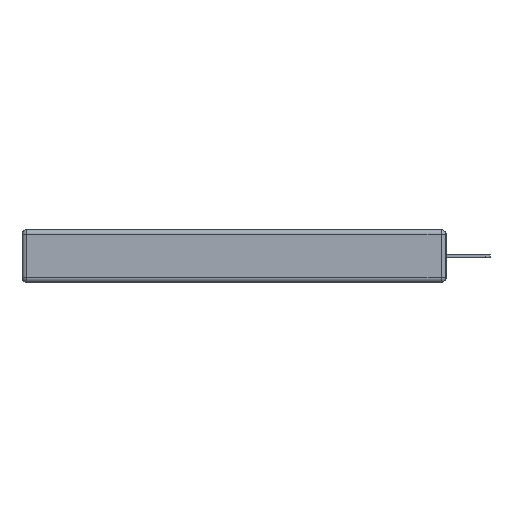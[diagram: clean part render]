
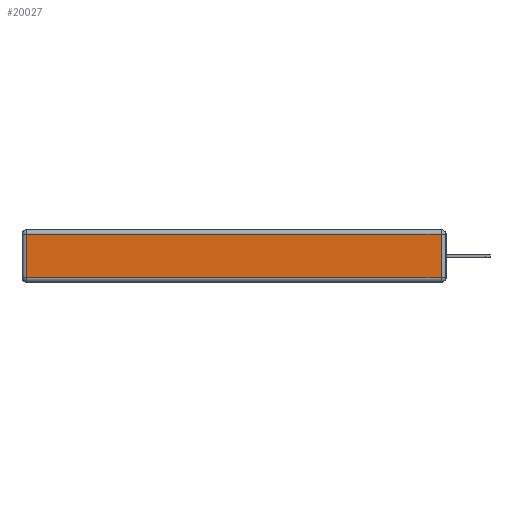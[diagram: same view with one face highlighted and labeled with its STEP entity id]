
A CAD part, left-side view. The second image highlights one B-rep face of the part: STEP entity #20027.
In plain terms, the highlighted planar face has unit normal (-1, 0, 0).
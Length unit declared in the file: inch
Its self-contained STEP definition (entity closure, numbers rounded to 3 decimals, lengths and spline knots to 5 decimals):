
#737 = VERTEX_POINT ( 'NONE', #9915 ) ;
#1229 = DIRECTION ( 'NONE',  ( 0., 0., -1. ) ) ;
#2094 = CARTESIAN_POINT ( 'NONE',  ( 0., 0.03, -0.313 ) ) ;
#2877 = VERTEX_POINT ( 'NONE', #12601 ) ;
#3298 = LINE ( 'NONE', #4908, #15899 ) ;
#4462 = ORIENTED_EDGE ( 'NONE', *, *, #9587, .T. ) ;
#4630 = AXIS2_PLACEMENT_3D ( 'NONE', #5800, #20575, #10771 ) ;
#4908 = CARTESIAN_POINT ( 'NONE',  ( 0., 2.75, -0.03 ) ) ;
#5800 = CARTESIAN_POINT ( 'NONE',  ( 0., 0., -0.343 ) ) ;
#6004 = VECTOR ( 'NONE', #14688, 39.37008 ) ;
#6624 = VECTOR ( 'NONE', #1229, 39.37008 ) ;
#7088 = ORIENTED_EDGE ( 'NONE', *, *, #15005, .T. ) ;
#7971 = ORIENTED_EDGE ( 'NONE', *, *, #14155, .T. ) ;
#8045 = EDGE_LOOP ( 'NONE', ( #7971, #7088, #4462, #19227 ) ) ;
#9132 = PLANE ( 'NONE',  #4630 ) ;
#9587 = EDGE_CURVE ( 'NONE', #2877, #21043, #3298, .T. ) ;
#9915 = CARTESIAN_POINT ( 'NONE',  ( 0., 2.72, -0.313 ) ) ;
#10771 = DIRECTION ( 'NONE',  ( 0., 0., 1. ) ) ;
#11085 = FACE_OUTER_BOUND ( 'NONE', #8045, .T. ) ;
#12520 = CARTESIAN_POINT ( 'NONE',  ( 0., 0., -0.313 ) ) ;
#12601 = CARTESIAN_POINT ( 'NONE',  ( 0., 0.03, -0.03 ) ) ;
#12694 = EDGE_CURVE ( 'NONE', #21043, #737, #19724, .T. ) ;
#12705 = CARTESIAN_POINT ( 'NONE',  ( 0., 2.72, -0.343 ) ) ;
#13309 = VERTEX_POINT ( 'NONE', #2094 ) ;
#13786 = LINE ( 'NONE', #12520, #17615 ) ;
#14155 = EDGE_CURVE ( 'NONE', #737, #13309, #13786, .T. ) ;
#14192 = DIRECTION ( 'NONE',  ( 0., -1., 0. ) ) ;
#14258 = LINE ( 'NONE', #19597, #6004 ) ;
#14688 = DIRECTION ( 'NONE',  ( 0., 0., 1. ) ) ;
#15005 = EDGE_CURVE ( 'NONE', #13309, #2877, #14258, .T. ) ;
#15089 = CARTESIAN_POINT ( 'NONE',  ( 0., 2.72, -0.03 ) ) ;
#15899 = VECTOR ( 'NONE', #18038, 39.37008 ) ;
#17615 = VECTOR ( 'NONE', #14192, 39.37008 ) ;
#18038 = DIRECTION ( 'NONE',  ( 0., 1., 0. ) ) ;
#19227 = ORIENTED_EDGE ( 'NONE', *, *, #12694, .T. ) ;
#19597 = CARTESIAN_POINT ( 'NONE',  ( 0., 0.03, -0.343 ) ) ;
#19724 = LINE ( 'NONE', #12705, #6624 ) ;
#20027 = ADVANCED_FACE ( 'NONE', ( #11085 ), #9132, .T. ) ;
#20575 = DIRECTION ( 'NONE',  ( -1., 0., 0. ) ) ;
#21043 = VERTEX_POINT ( 'NONE', #15089 ) ;
